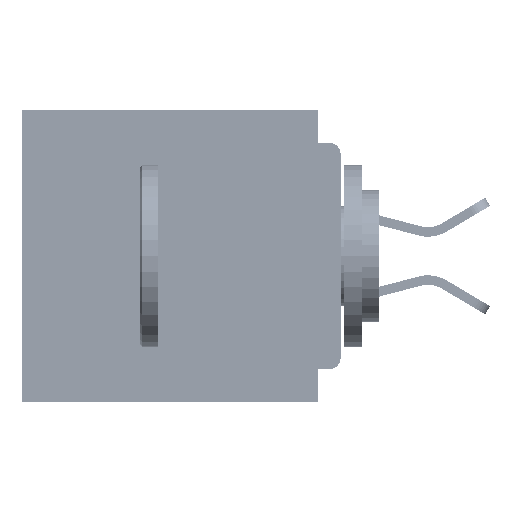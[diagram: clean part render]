
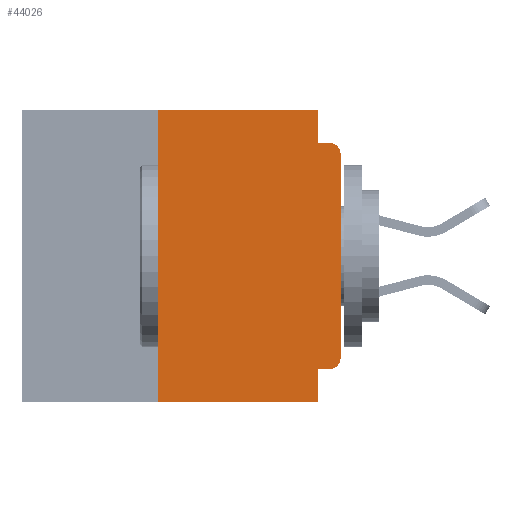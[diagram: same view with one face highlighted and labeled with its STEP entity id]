
A CAD part, left-side view. The second image highlights one B-rep face of the part: STEP entity #44026.
In plain terms, the highlighted planar face has unit normal (-1, 0, 0).
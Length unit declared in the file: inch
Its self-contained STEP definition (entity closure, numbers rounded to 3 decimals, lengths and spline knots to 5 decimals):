
#736 = VECTOR ( 'NONE', #6659, 39.37008 ) ;
#1685 = ORIENTED_EDGE ( 'NONE', *, *, #54587, .T. ) ;
#2491 = CARTESIAN_POINT ( 'NONE',  ( 0., 0., -0.06 ) ) ;
#2659 = ORIENTED_EDGE ( 'NONE', *, *, #29607, .T. ) ;
#2695 = CARTESIAN_POINT ( 'NONE',  ( 0., 0.437, 0. ) ) ;
#3738 = CARTESIAN_POINT ( 'NONE',  ( 0., 0., -0.045 ) ) ;
#3787 = VERTEX_POINT ( 'NONE', #38256 ) ;
#3853 = VERTEX_POINT ( 'NONE', #9449 ) ;
#4118 = VECTOR ( 'NONE', #47722, 39.37008 ) ;
#4679 = CARTESIAN_POINT ( 'NONE',  ( 0., 0.031, -0.045 ) ) ;
#4807 = CARTESIAN_POINT ( 'NONE',  ( 0., 0.437, -0.4 ) ) ;
#5084 = AXIS2_PLACEMENT_3D ( 'NONE', #2695, #36953, #7675 ) ;
#5152 = DIRECTION ( 'NONE',  ( 0., 1., 0. ) ) ;
#5630 = EDGE_CURVE ( 'NONE', #51077, #58997, #28975, .T. ) ;
#6459 = ORIENTED_EDGE ( 'NONE', *, *, #43335, .F. ) ;
#6659 = DIRECTION ( 'NONE',  ( 0., 0., 1. ) ) ;
#6974 = DIRECTION ( 'NONE',  ( 0., -1., 0. ) ) ;
#7675 = DIRECTION ( 'NONE',  ( 0., 0., -1. ) ) ;
#9449 = CARTESIAN_POINT ( 'NONE',  ( 0., 0.031, 0. ) ) ;
#9695 = EDGE_LOOP ( 'NONE', ( #46501, #45220, #41116, #44756, #14473, #6459, #2659, #41631, #16305, #1685 ) ) ;
#9827 = VERTEX_POINT ( 'NONE', #4679 ) ;
#9955 = CARTESIAN_POINT ( 'NONE',  ( 0., 0., 0. ) ) ;
#10102 = VERTEX_POINT ( 'NONE', #36311 ) ;
#11016 = EDGE_CURVE ( 'NONE', #3853, #9827, #56411, .T. ) ;
#13041 = FACE_OUTER_BOUND ( 'NONE', #9695, .T. ) ;
#13257 = CARTESIAN_POINT ( 'NONE',  ( 0., 0.015, -0.045 ) ) ;
#13915 = LINE ( 'NONE', #60049, #736 ) ;
#14336 = VERTEX_POINT ( 'NONE', #26497 ) ;
#14473 = ORIENTED_EDGE ( 'NONE', *, *, #46444, .F. ) ;
#15323 = CIRCLE ( 'NONE', #29121, 0.015 ) ;
#16305 = ORIENTED_EDGE ( 'NONE', *, *, #43164, .F. ) ;
#16876 = CARTESIAN_POINT ( 'NONE',  ( 0., 0.031, 0. ) ) ;
#19415 = DIRECTION ( 'NONE',  ( -1., 0., 0. ) ) ;
#19721 = DIRECTION ( 'NONE',  ( 0., -1., 0. ) ) ;
#20069 = EDGE_CURVE ( 'NONE', #45056, #14336, #24027, .T. ) ;
#21450 = DIRECTION ( 'NONE',  ( -1., 0., 0. ) ) ;
#21603 = CARTESIAN_POINT ( 'NONE',  ( 0., 0.437, 0. ) ) ;
#24027 = LINE ( 'NONE', #35746, #48276 ) ;
#26497 = CARTESIAN_POINT ( 'NONE',  ( 0., 0.031, -0.4 ) ) ;
#27668 = VECTOR ( 'NONE', #19721, 39.37008 ) ;
#27970 = VERTEX_POINT ( 'NONE', #49432 ) ;
#28975 = LINE ( 'NONE', #9955, #43468 ) ;
#29121 = AXIS2_PLACEMENT_3D ( 'NONE', #48483, #19415, #53328 ) ;
#29607 = EDGE_CURVE ( 'NONE', #10102, #14336, #40623, .T. ) ;
#32041 = PLANE ( 'NONE',  #5084 ) ;
#32141 = VECTOR ( 'NONE', #50802, 39.37008 ) ;
#34312 = EDGE_CURVE ( 'NONE', #9827, #62003, #55976, .T. ) ;
#35746 = CARTESIAN_POINT ( 'NONE',  ( 0., 0.031, -0.4 ) ) ;
#36311 = CARTESIAN_POINT ( 'NONE',  ( 0., 0.25, -0.4 ) ) ;
#36953 = DIRECTION ( 'NONE',  ( 1., 0., 0. ) ) ;
#38256 = CARTESIAN_POINT ( 'NONE',  ( 0., 0.25, 0. ) ) ;
#40035 = CARTESIAN_POINT ( 'NONE',  ( 0., 0.031, -0.355 ) ) ;
#40623 = LINE ( 'NONE', #4807, #27668 ) ;
#40681 = DIRECTION ( 'NONE',  ( 0., 0., -1. ) ) ;
#41116 = ORIENTED_EDGE ( 'NONE', *, *, #34312, .F. ) ;
#41631 = ORIENTED_EDGE ( 'NONE', *, *, #20069, .F. ) ;
#43164 = EDGE_CURVE ( 'NONE', #27970, #45056, #47564, .T. ) ;
#43335 = EDGE_CURVE ( 'NONE', #10102, #3787, #13915, .T. ) ;
#43468 = VECTOR ( 'NONE', #58422, 39.37008 ) ;
#44026 = ADVANCED_FACE ( 'NONE', ( #13041 ), #32041, .F. ) ;
#44740 = VECTOR ( 'NONE', #6974, 39.37008 ) ;
#44756 = ORIENTED_EDGE ( 'NONE', *, *, #11016, .F. ) ;
#45056 = VERTEX_POINT ( 'NONE', #40035 ) ;
#45220 = ORIENTED_EDGE ( 'NONE', *, *, #49169, .T. ) ;
#46052 = VECTOR ( 'NONE', #5152, 39.37008 ) ;
#46444 = EDGE_CURVE ( 'NONE', #3787, #3853, #57568, .T. ) ;
#46487 = CARTESIAN_POINT ( 'NONE',  ( 0., 0., -0.34 ) ) ;
#46501 = ORIENTED_EDGE ( 'NONE', *, *, #5630, .T. ) ;
#47564 = LINE ( 'NONE', #58616, #46052 ) ;
#47722 = DIRECTION ( 'NONE',  ( 0., -1., 0. ) ) ;
#48276 = VECTOR ( 'NONE', #40681, 39.37008 ) ;
#48483 = CARTESIAN_POINT ( 'NONE',  ( 0., 0.015, -0.34 ) ) ;
#49169 = EDGE_CURVE ( 'NONE', #58997, #62003, #54424, .T. ) ;
#49432 = CARTESIAN_POINT ( 'NONE',  ( 0., 0.015, -0.355 ) ) ;
#50470 = CARTESIAN_POINT ( 'NONE',  ( 0., 0.015, -0.06 ) ) ;
#50802 = DIRECTION ( 'NONE',  ( 0., 0., -1. ) ) ;
#51077 = VERTEX_POINT ( 'NONE', #46487 ) ;
#53328 = DIRECTION ( 'NONE',  ( 0., 0., -1. ) ) ;
#54424 = CIRCLE ( 'NONE', #61567, 0.015 ) ;
#54587 = EDGE_CURVE ( 'NONE', #27970, #51077, #15323, .T. ) ;
#55333 = DIRECTION ( 'NONE',  ( 0., 0., -1. ) ) ;
#55976 = LINE ( 'NONE', #3738, #4118 ) ;
#56411 = LINE ( 'NONE', #16876, #32141 ) ;
#57568 = LINE ( 'NONE', #21603, #44740 ) ;
#58422 = DIRECTION ( 'NONE',  ( 0., 0., 1. ) ) ;
#58616 = CARTESIAN_POINT ( 'NONE',  ( 0., 0., -0.355 ) ) ;
#58997 = VERTEX_POINT ( 'NONE', #2491 ) ;
#60049 = CARTESIAN_POINT ( 'NONE',  ( 0., 0.25, -0.4 ) ) ;
#61567 = AXIS2_PLACEMENT_3D ( 'NONE', #50470, #21450, #55333 ) ;
#62003 = VERTEX_POINT ( 'NONE', #13257 ) ;
